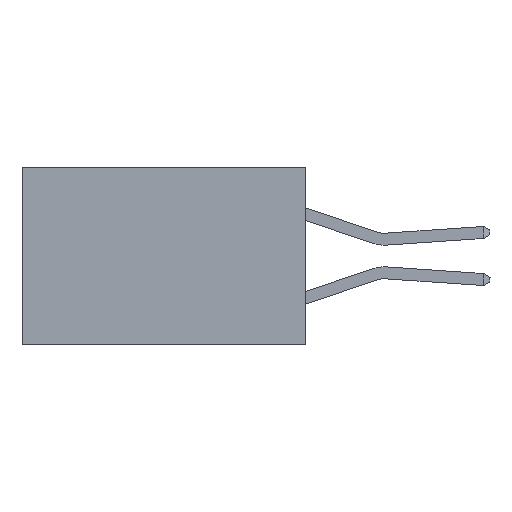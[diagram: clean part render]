
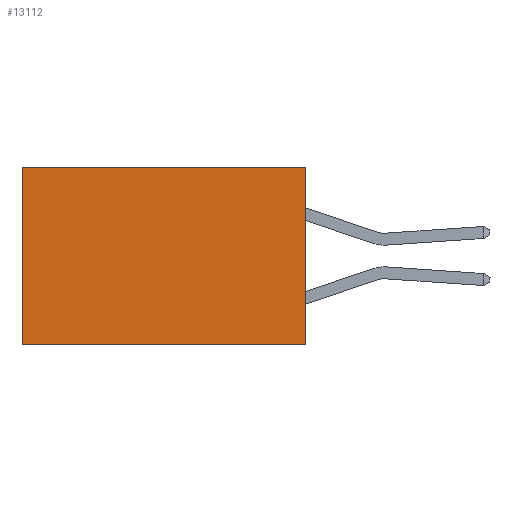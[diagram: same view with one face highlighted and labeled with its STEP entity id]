
A CAD part, left-side view. The second image highlights one B-rep face of the part: STEP entity #13112.
In plain terms, the highlighted planar face has unit normal (-1, 0, 0).
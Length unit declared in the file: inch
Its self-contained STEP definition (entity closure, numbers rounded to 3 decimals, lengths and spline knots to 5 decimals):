
#1484 = VECTOR ( 'NONE', #4060, 39.37008 ) ;
#1996 = CARTESIAN_POINT ( 'NONE',  ( 0.277, 0., -0.37 ) ) ;
#2588 = DIRECTION ( 'NONE',  ( 1., 0., 0. ) ) ;
#2888 = CARTESIAN_POINT ( 'NONE',  ( 0.277, 0., 0. ) ) ;
#3451 = CARTESIAN_POINT ( 'NONE',  ( 0.277, 0.59, 0. ) ) ;
#4060 = DIRECTION ( 'NONE',  ( 0., 1., 0. ) ) ;
#5695 = LINE ( 'NONE', #22536, #19695 ) ;
#6871 = LINE ( 'NONE', #1996, #1484 ) ;
#7188 = DIRECTION ( 'NONE',  ( 0., 0., -1. ) ) ;
#8599 = EDGE_CURVE ( 'NONE', #17524, #18399, #11903, .T. ) ;
#11162 = VERTEX_POINT ( 'NONE', #12901 ) ;
#11903 = LINE ( 'NONE', #20216, #21779 ) ;
#12749 = ORIENTED_EDGE ( 'NONE', *, *, #18348, .T. ) ;
#12901 = CARTESIAN_POINT ( 'NONE',  ( 0.277, 0.59, -0.37 ) ) ;
#13112 = ADVANCED_FACE ( 'NONE', ( #25307 ), #18557, .F. ) ;
#14654 = CARTESIAN_POINT ( 'NONE',  ( 0.277, 0., -0.37 ) ) ;
#15070 = CARTESIAN_POINT ( 'NONE',  ( 0.277, 0.59, -0.37 ) ) ;
#16222 = ORIENTED_EDGE ( 'NONE', *, *, #8599, .F. ) ;
#16372 = VECTOR ( 'NONE', #7188, 39.37008 ) ;
#16660 = DIRECTION ( 'NONE',  ( 0., 0., -1. ) ) ;
#17031 = DIRECTION ( 'NONE',  ( 0., 0., -1. ) ) ;
#17342 = CARTESIAN_POINT ( 'NONE',  ( 0.277, 0., -0.37 ) ) ;
#17524 = VERTEX_POINT ( 'NONE', #2888 ) ;
#18348 = EDGE_CURVE ( 'NONE', #19105, #11162, #21559, .T. ) ;
#18399 = VERTEX_POINT ( 'NONE', #17342 ) ;
#18557 = PLANE ( 'NONE',  #22010 ) ;
#19105 = VERTEX_POINT ( 'NONE', #3451 ) ;
#19511 = EDGE_CURVE ( 'NONE', #17524, #19105, #5695, .T. ) ;
#19695 = VECTOR ( 'NONE', #24492, 39.37008 ) ;
#20216 = CARTESIAN_POINT ( 'NONE',  ( 0.277, 0., -0.37 ) ) ;
#20772 = EDGE_CURVE ( 'NONE', #18399, #11162, #6871, .T. ) ;
#20940 = EDGE_LOOP ( 'NONE', ( #12749, #22293, #16222, #25636 ) ) ;
#21559 = LINE ( 'NONE', #15070, #16372 ) ;
#21779 = VECTOR ( 'NONE', #17031, 39.37008 ) ;
#22010 = AXIS2_PLACEMENT_3D ( 'NONE', #14654, #2588, #16660 ) ;
#22293 = ORIENTED_EDGE ( 'NONE', *, *, #20772, .F. ) ;
#22536 = CARTESIAN_POINT ( 'NONE',  ( 0.277, 0., 0. ) ) ;
#24492 = DIRECTION ( 'NONE',  ( 0., 1., 0. ) ) ;
#25307 = FACE_OUTER_BOUND ( 'NONE', #20940, .T. ) ;
#25636 = ORIENTED_EDGE ( 'NONE', *, *, #19511, .T. ) ;
